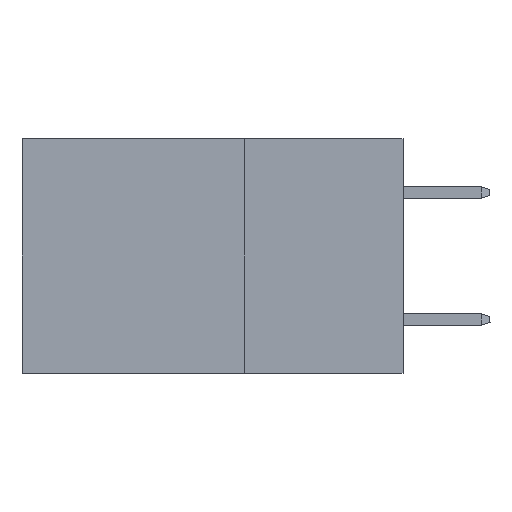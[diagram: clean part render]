
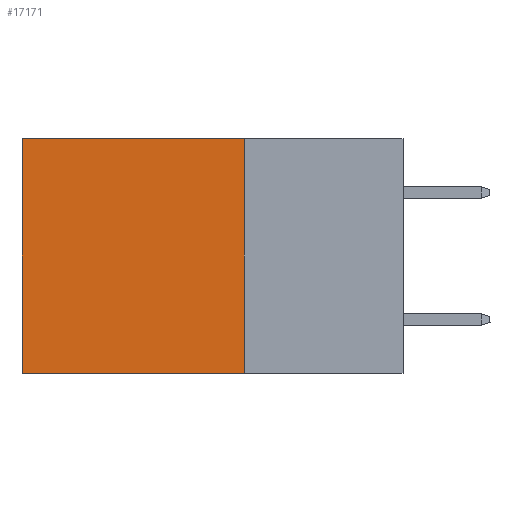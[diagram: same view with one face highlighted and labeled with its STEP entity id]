
A CAD part, left-side view. The second image highlights one B-rep face of the part: STEP entity #17171.
In plain terms, the highlighted planar face has unit normal (-1, 0, 0).
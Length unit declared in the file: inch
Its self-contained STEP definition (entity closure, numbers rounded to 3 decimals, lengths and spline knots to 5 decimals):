
#194 = LINE ( 'NONE', #16203, #19358 ) ;
#1192 = ORIENTED_EDGE ( 'NONE', *, *, #20753, .F. ) ;
#2354 = VERTEX_POINT ( 'NONE', #17946 ) ;
#3203 = DIRECTION ( 'NONE',  ( 0., 1., 0. ) ) ;
#4802 = PLANE ( 'NONE',  #5829 ) ;
#5829 = AXIS2_PLACEMENT_3D ( 'NONE', #12660, #6774, #23169 ) ;
#6029 = ORIENTED_EDGE ( 'NONE', *, *, #22792, .F. ) ;
#6774 = DIRECTION ( 'NONE',  ( 1., 0., 0. ) ) ;
#9272 = LINE ( 'NONE', #15309, #19600 ) ;
#9526 = VERTEX_POINT ( 'NONE', #23859 ) ;
#9891 = VERTEX_POINT ( 'NONE', #18177 ) ;
#11433 = CARTESIAN_POINT ( 'NONE',  ( 0.2875, 0.25, -0.37 ) ) ;
#12660 = CARTESIAN_POINT ( 'NONE',  ( 0.2875, 0.25, 0. ) ) ;
#13294 = VERTEX_POINT ( 'NONE', #21286 ) ;
#13774 = DIRECTION ( 'NONE',  ( 0., 1., 0. ) ) ;
#14643 = FACE_OUTER_BOUND ( 'NONE', #24257, .T. ) ;
#15087 = VECTOR ( 'NONE', #13774, 39.37008 ) ;
#15309 = CARTESIAN_POINT ( 'NONE',  ( 0.2875, 0.6, 0. ) ) ;
#15447 = EDGE_CURVE ( 'NONE', #9891, #2354, #9272, .T. ) ;
#16203 = CARTESIAN_POINT ( 'NONE',  ( 0.2875, 0.25, 0. ) ) ;
#17171 = ADVANCED_FACE ( 'NONE', ( #14643 ), #4802, .F. ) ;
#17946 = CARTESIAN_POINT ( 'NONE',  ( 0.2875, 0.6, -0.37 ) ) ;
#18177 = CARTESIAN_POINT ( 'NONE',  ( 0.2875, 0.6, 0. ) ) ;
#18553 = VECTOR ( 'NONE', #3203, 39.37008 ) ;
#19358 = VECTOR ( 'NONE', #24206, 39.37008 ) ;
#19600 = VECTOR ( 'NONE', #20962, 39.37008 ) ;
#20753 = EDGE_CURVE ( 'NONE', #9526, #2354, #25588, .T. ) ;
#20962 = DIRECTION ( 'NONE',  ( 0., 0., -1. ) ) ;
#21191 = LINE ( 'NONE', #21571, #18553 ) ;
#21286 = CARTESIAN_POINT ( 'NONE',  ( 0.2875, 0.25, 0. ) ) ;
#21571 = CARTESIAN_POINT ( 'NONE',  ( 0.2875, 0.25, 0. ) ) ;
#22021 = ORIENTED_EDGE ( 'NONE', *, *, #23099, .T. ) ;
#22783 = ORIENTED_EDGE ( 'NONE', *, *, #15447, .T. ) ;
#22792 = EDGE_CURVE ( 'NONE', #13294, #9526, #194, .T. ) ;
#23099 = EDGE_CURVE ( 'NONE', #13294, #9891, #21191, .T. ) ;
#23169 = DIRECTION ( 'NONE',  ( 0., 0., -1. ) ) ;
#23859 = CARTESIAN_POINT ( 'NONE',  ( 0.2875, 0.25, -0.37 ) ) ;
#24206 = DIRECTION ( 'NONE',  ( 0., 0., -1. ) ) ;
#24257 = EDGE_LOOP ( 'NONE', ( #22783, #1192, #6029, #22021 ) ) ;
#25588 = LINE ( 'NONE', #11433, #15087 ) ;
